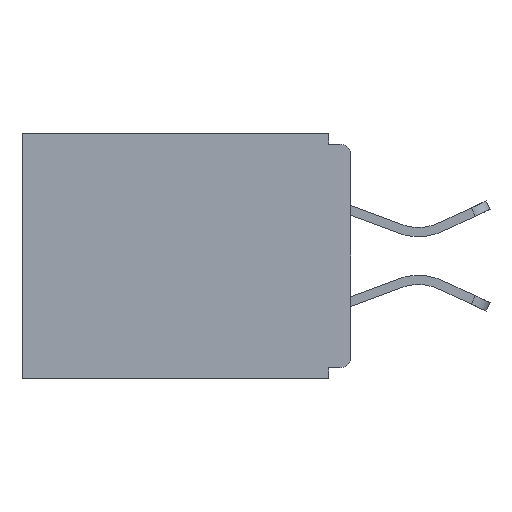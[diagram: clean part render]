
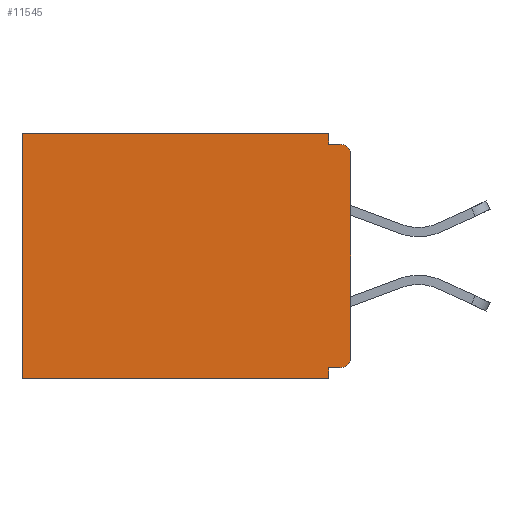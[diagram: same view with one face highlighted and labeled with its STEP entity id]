
A CAD part, left-side view. The second image highlights one B-rep face of the part: STEP entity #11545.
In plain terms, the highlighted planar face has unit normal (-1, 0, 0).
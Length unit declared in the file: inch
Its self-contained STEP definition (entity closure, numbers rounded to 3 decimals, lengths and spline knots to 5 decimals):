
#69 = DIRECTION ( 'NONE',  ( 0., 0., -1. ) ) ;
#282 = CARTESIAN_POINT ( 'NONE',  ( 0.298, 0.015, -0.313 ) ) ;
#371 = LINE ( 'NONE', #3055, #799 ) ;
#519 = CARTESIAN_POINT ( 'NONE',  ( 0.298, 0.46, 0. ) ) ;
#799 = VECTOR ( 'NONE', #8175, 39.37008 ) ;
#937 = CARTESIAN_POINT ( 'NONE',  ( 0.298, 0.031, -0.015 ) ) ;
#948 = DIRECTION ( 'NONE',  ( 0., 0., -1. ) ) ;
#968 = LINE ( 'NONE', #9778, #3301 ) ;
#1530 = EDGE_CURVE ( 'NONE', #14297, #15041, #968, .T. ) ;
#2096 = AXIS2_PLACEMENT_3D ( 'NONE', #14801, #14735, #10637 ) ;
#2323 = VERTEX_POINT ( 'NONE', #16018 ) ;
#2359 = ORIENTED_EDGE ( 'NONE', *, *, #17201, .F. ) ;
#2595 = VECTOR ( 'NONE', #6571, 39.37008 ) ;
#2652 = ORIENTED_EDGE ( 'NONE', *, *, #8287, .F. ) ;
#2915 = CARTESIAN_POINT ( 'NONE',  ( 0.298, 0.015, -0.015 ) ) ;
#3055 = CARTESIAN_POINT ( 'NONE',  ( 0.298, 0., -0.343 ) ) ;
#3064 = ORIENTED_EDGE ( 'NONE', *, *, #1530, .F. ) ;
#3137 = DIRECTION ( 'NONE',  ( 0., 0., -1. ) ) ;
#3166 = CARTESIAN_POINT ( 'NONE',  ( 0.298, 0.031, -0.343 ) ) ;
#3279 = FACE_OUTER_BOUND ( 'NONE', #12764, .T. ) ;
#3301 = VECTOR ( 'NONE', #16694, 39.37008 ) ;
#3501 = DIRECTION ( 'NONE',  ( 1., 0., 0. ) ) ;
#3684 = CARTESIAN_POINT ( 'NONE',  ( 0.298, 0., 0. ) ) ;
#3802 = EDGE_CURVE ( 'NONE', #2323, #11798, #14687, .T. ) ;
#3969 = CIRCLE ( 'NONE', #9368, 0.015 ) ;
#4150 = VERTEX_POINT ( 'NONE', #16862 ) ;
#4204 = DIRECTION ( 'NONE',  ( -1., 0., 0. ) ) ;
#4456 = CARTESIAN_POINT ( 'NONE',  ( 0.298, 0.46, -0.343 ) ) ;
#5146 = LINE ( 'NONE', #6266, #12775 ) ;
#5348 = CARTESIAN_POINT ( 'NONE',  ( 0.298, 0., 0. ) ) ;
#5410 = CARTESIAN_POINT ( 'NONE',  ( 0.298, 0., 0. ) ) ;
#5618 = LINE ( 'NONE', #5410, #14737 ) ;
#6266 = CARTESIAN_POINT ( 'NONE',  ( 0.298, 0., -0.015 ) ) ;
#6268 = CARTESIAN_POINT ( 'NONE',  ( 0.298, 0., -0.313 ) ) ;
#6571 = DIRECTION ( 'NONE',  ( 0., 1., 0. ) ) ;
#6742 = CARTESIAN_POINT ( 'NONE',  ( 0.298, 0.031, -0.328 ) ) ;
#7029 = DIRECTION ( 'NONE',  ( 0., 0., -1. ) ) ;
#7338 = DIRECTION ( 'NONE',  ( 0., 0., -1. ) ) ;
#7421 = VERTEX_POINT ( 'NONE', #4456 ) ;
#7473 = CARTESIAN_POINT ( 'NONE',  ( 0.298, 0.031, 0. ) ) ;
#7997 = ORIENTED_EDGE ( 'NONE', *, *, #11396, .F. ) ;
#8175 = DIRECTION ( 'NONE',  ( 0., 1., 0. ) ) ;
#8287 = EDGE_CURVE ( 'NONE', #4150, #16057, #16291, .T. ) ;
#8652 = VERTEX_POINT ( 'NONE', #10322 ) ;
#8870 = ORIENTED_EDGE ( 'NONE', *, *, #10784, .T. ) ;
#9368 = AXIS2_PLACEMENT_3D ( 'NONE', #282, #4204, #7029 ) ;
#9502 = EDGE_CURVE ( 'NONE', #2323, #16057, #3969, .T. ) ;
#9778 = CARTESIAN_POINT ( 'NONE',  ( 0.298, 0.031, -0.343 ) ) ;
#10258 = VECTOR ( 'NONE', #3137, 39.37008 ) ;
#10322 = CARTESIAN_POINT ( 'NONE',  ( 0.298, 0.031, -0.343 ) ) ;
#10611 = ORIENTED_EDGE ( 'NONE', *, *, #14071, .T. ) ;
#10637 = DIRECTION ( 'NONE',  ( 0., 0., -1. ) ) ;
#10784 = EDGE_CURVE ( 'NONE', #14297, #14215, #5618, .T. ) ;
#11246 = CIRCLE ( 'NONE', #2096, 0.015 ) ;
#11310 = VERTEX_POINT ( 'NONE', #2915 ) ;
#11396 = EDGE_CURVE ( 'NONE', #11798, #8652, #15972, .T. ) ;
#11544 = ORIENTED_EDGE ( 'NONE', *, *, #16140, .T. ) ;
#11545 = ADVANCED_FACE ( 'NONE', ( #3279 ), #15812, .F. ) ;
#11568 = AXIS2_PLACEMENT_3D ( 'NONE', #3684, #3501, #948 ) ;
#11763 = CARTESIAN_POINT ( 'NONE',  ( 0.298, 0.46, 0. ) ) ;
#11798 = VERTEX_POINT ( 'NONE', #6742 ) ;
#12675 = VECTOR ( 'NONE', #69, 39.37008 ) ;
#12678 = ORIENTED_EDGE ( 'NONE', *, *, #3802, .F. ) ;
#12764 = EDGE_LOOP ( 'NONE', ( #11544, #15217, #3064, #8870, #10611, #2359, #7997, #12678, #16358, #2652 ) ) ;
#12775 = VECTOR ( 'NONE', #14443, 39.37008 ) ;
#13120 = EDGE_CURVE ( 'NONE', #15041, #11310, #5146, .T. ) ;
#14071 = EDGE_CURVE ( 'NONE', #14215, #7421, #17230, .T. ) ;
#14215 = VERTEX_POINT ( 'NONE', #11763 ) ;
#14297 = VERTEX_POINT ( 'NONE', #7473 ) ;
#14443 = DIRECTION ( 'NONE',  ( 0., -1., 0. ) ) ;
#14687 = LINE ( 'NONE', #14691, #2595 ) ;
#14691 = CARTESIAN_POINT ( 'NONE',  ( 0.298, 0., -0.328 ) ) ;
#14735 = DIRECTION ( 'NONE',  ( -1., 0., 0. ) ) ;
#14737 = VECTOR ( 'NONE', #14906, 39.37008 ) ;
#14801 = CARTESIAN_POINT ( 'NONE',  ( 0.298, 0.015, -0.03 ) ) ;
#14906 = DIRECTION ( 'NONE',  ( 0., 1., 0. ) ) ;
#15041 = VERTEX_POINT ( 'NONE', #937 ) ;
#15217 = ORIENTED_EDGE ( 'NONE', *, *, #13120, .F. ) ;
#15782 = VECTOR ( 'NONE', #7338, 39.37008 ) ;
#15812 = PLANE ( 'NONE',  #11568 ) ;
#15972 = LINE ( 'NONE', #3166, #15782 ) ;
#16018 = CARTESIAN_POINT ( 'NONE',  ( 0.298, 0.015, -0.328 ) ) ;
#16057 = VERTEX_POINT ( 'NONE', #6268 ) ;
#16140 = EDGE_CURVE ( 'NONE', #4150, #11310, #11246, .T. ) ;
#16291 = LINE ( 'NONE', #5348, #12675 ) ;
#16358 = ORIENTED_EDGE ( 'NONE', *, *, #9502, .T. ) ;
#16694 = DIRECTION ( 'NONE',  ( 0., 0., -1. ) ) ;
#16862 = CARTESIAN_POINT ( 'NONE',  ( 0.298, 0., -0.03 ) ) ;
#17201 = EDGE_CURVE ( 'NONE', #8652, #7421, #371, .T. ) ;
#17230 = LINE ( 'NONE', #519, #10258 ) ;
